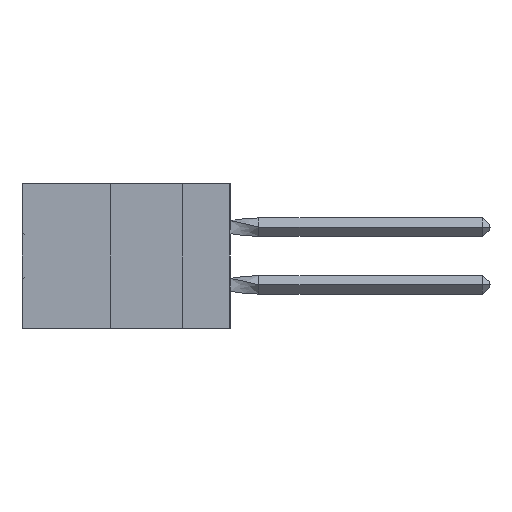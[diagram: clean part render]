
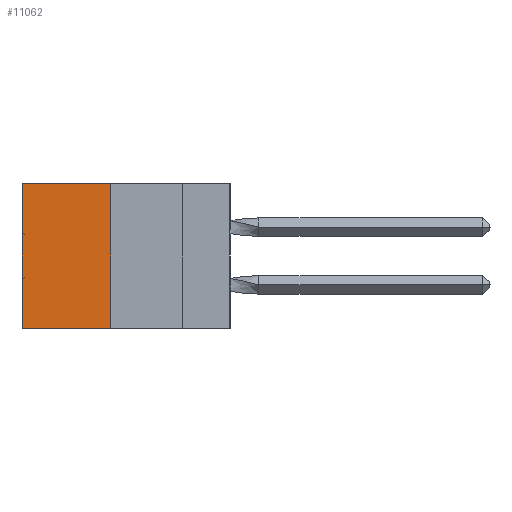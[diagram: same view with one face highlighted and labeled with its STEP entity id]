
A CAD part, left-side view. The second image highlights one B-rep face of the part: STEP entity #11062.
In plain terms, the highlighted planar face has unit normal (-1, 0, 0).
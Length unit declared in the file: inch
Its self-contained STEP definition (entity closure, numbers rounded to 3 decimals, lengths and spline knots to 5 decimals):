
#1 = CARTESIAN_POINT ( 'NONE',  ( 0.305, 0.72, -0.5 ) ) ;
#730 = CARTESIAN_POINT ( 'NONE',  ( 0.305, 0.413, -0.5 ) ) ;
#1632 = LINE ( 'NONE', #15507, #7110 ) ;
#4947 = EDGE_LOOP ( 'NONE', ( #29440, #21319, #16681, #13924 ) ) ;
#7110 = VECTOR ( 'NONE', #19692, 39.37008 ) ;
#9285 = CARTESIAN_POINT ( 'NONE',  ( 0.305, 0.413, 0. ) ) ;
#9340 = VERTEX_POINT ( 'NONE', #46178 ) ;
#11060 = EDGE_CURVE ( 'NONE', #21949, #9340, #37451, .T. ) ;
#11062 = ADVANCED_FACE ( 'NONE', ( #19008 ), #15804, .F. ) ;
#11401 = CARTESIAN_POINT ( 'NONE',  ( 0.305, 0.413, -0.5 ) ) ;
#13541 = EDGE_CURVE ( 'NONE', #43480, #20684, #1632, .T. ) ;
#13924 = ORIENTED_EDGE ( 'NONE', *, *, #13541, .T. ) ;
#15040 = DIRECTION ( 'NONE',  ( 0., 0., -1. ) ) ;
#15507 = CARTESIAN_POINT ( 'NONE',  ( 0.305, 0.413, 0. ) ) ;
#15613 = CARTESIAN_POINT ( 'NONE',  ( 0.305, 0.413, -0.5 ) ) ;
#15804 = PLANE ( 'NONE',  #46024 ) ;
#16681 = ORIENTED_EDGE ( 'NONE', *, *, #52025, .F. ) ;
#17477 = LINE ( 'NONE', #1, #36559 ) ;
#19008 = FACE_OUTER_BOUND ( 'NONE', #4947, .T. ) ;
#19026 = DIRECTION ( 'NONE',  ( 0., 0., -1. ) ) ;
#19692 = DIRECTION ( 'NONE',  ( 0., 1., 0. ) ) ;
#20684 = VERTEX_POINT ( 'NONE', #25569 ) ;
#21319 = ORIENTED_EDGE ( 'NONE', *, *, #11060, .F. ) ;
#21949 = VERTEX_POINT ( 'NONE', #730 ) ;
#25053 = VECTOR ( 'NONE', #19026, 39.37008 ) ;
#25569 = CARTESIAN_POINT ( 'NONE',  ( 0.305, 0.72, 0. ) ) ;
#25938 = DIRECTION ( 'NONE',  ( 0., 0., -1. ) ) ;
#29440 = ORIENTED_EDGE ( 'NONE', *, *, #53044, .T. ) ;
#31898 = LINE ( 'NONE', #54424, #25053 ) ;
#36559 = VECTOR ( 'NONE', #25938, 39.37008 ) ;
#37451 = LINE ( 'NONE', #15613, #40887 ) ;
#40887 = VECTOR ( 'NONE', #41947, 39.37008 ) ;
#41947 = DIRECTION ( 'NONE',  ( 0., 1., 0. ) ) ;
#43480 = VERTEX_POINT ( 'NONE', #9285 ) ;
#46024 = AXIS2_PLACEMENT_3D ( 'NONE', #11401, #46377, #15040 ) ;
#46178 = CARTESIAN_POINT ( 'NONE',  ( 0.305, 0.72, -0.5 ) ) ;
#46377 = DIRECTION ( 'NONE',  ( 1., 0., 0. ) ) ;
#52025 = EDGE_CURVE ( 'NONE', #43480, #21949, #31898, .T. ) ;
#53044 = EDGE_CURVE ( 'NONE', #20684, #9340, #17477, .T. ) ;
#54424 = CARTESIAN_POINT ( 'NONE',  ( 0.305, 0.413, -0.5 ) ) ;
